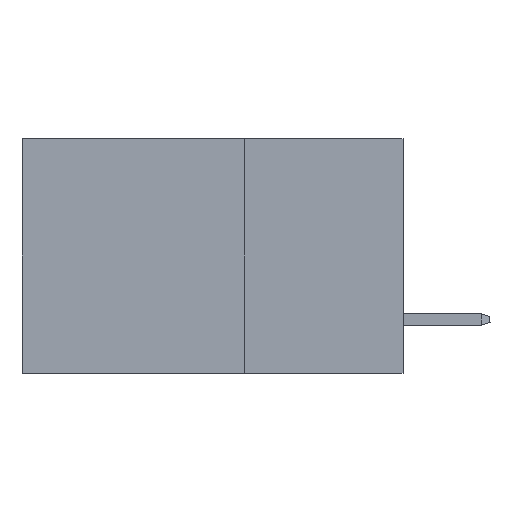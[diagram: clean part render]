
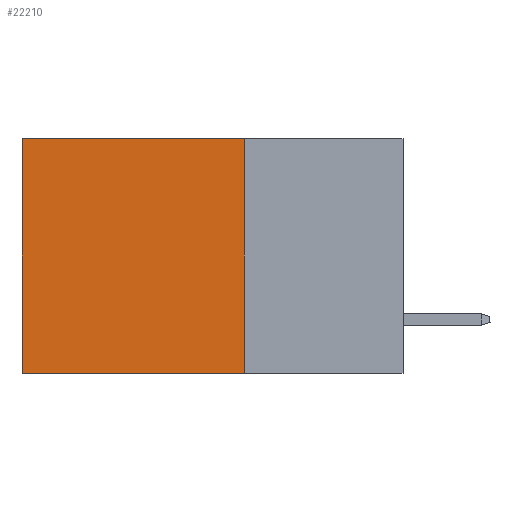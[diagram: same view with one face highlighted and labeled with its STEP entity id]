
A CAD part, left-side view. The second image highlights one B-rep face of the part: STEP entity #22210.
In plain terms, the highlighted planar face has unit normal (-1, 0, 0).
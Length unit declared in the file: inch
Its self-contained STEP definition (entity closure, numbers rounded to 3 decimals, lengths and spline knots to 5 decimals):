
#967 = DIRECTION ( 'NONE',  ( 0., 1., 0. ) ) ;
#1130 = EDGE_CURVE ( 'NONE', #6470, #13392, #18044, .T. ) ;
#1162 = CARTESIAN_POINT ( 'NONE',  ( 0.2875, 0.25, -0.37 ) ) ;
#1659 = CARTESIAN_POINT ( 'NONE',  ( 0.2875, 0.25, -0.37 ) ) ;
#2454 = VERTEX_POINT ( 'NONE', #1659 ) ;
#2565 = ORIENTED_EDGE ( 'NONE', *, *, #24105, .T. ) ;
#3547 = AXIS2_PLACEMENT_3D ( 'NONE', #9867, #39297, #10278 ) ;
#4322 = CARTESIAN_POINT ( 'NONE',  ( 0.2875, 0.25, 0. ) ) ;
#4441 = LINE ( 'NONE', #20441, #12994 ) ;
#4744 = VECTOR ( 'NONE', #10909, 39.37008 ) ;
#6132 = EDGE_LOOP ( 'NONE', ( #20596, #29836, #34292, #2565 ) ) ;
#6470 = VERTEX_POINT ( 'NONE', #37804 ) ;
#7472 = DIRECTION ( 'NONE',  ( 0., 1., 0. ) ) ;
#9821 = EDGE_CURVE ( 'NONE', #29669, #2454, #4441, .T. ) ;
#9867 = CARTESIAN_POINT ( 'NONE',  ( 0.2875, 0.25, 0. ) ) ;
#10278 = DIRECTION ( 'NONE',  ( 0., 0., -1. ) ) ;
#10909 = DIRECTION ( 'NONE',  ( 0., 0., -1. ) ) ;
#12268 = VECTOR ( 'NONE', #7472, 39.37008 ) ;
#12994 = VECTOR ( 'NONE', #30110, 39.37008 ) ;
#13392 = VERTEX_POINT ( 'NONE', #24542 ) ;
#17405 = CARTESIAN_POINT ( 'NONE',  ( 0.2875, 0.25, 0. ) ) ;
#18044 = LINE ( 'NONE', #37199, #4744 ) ;
#20441 = CARTESIAN_POINT ( 'NONE',  ( 0.2875, 0.25, 0. ) ) ;
#20596 = ORIENTED_EDGE ( 'NONE', *, *, #1130, .T. ) ;
#21092 = VECTOR ( 'NONE', #967, 39.37008 ) ;
#22210 = ADVANCED_FACE ( 'NONE', ( #35292 ), #32564, .F. ) ;
#22814 = EDGE_CURVE ( 'NONE', #2454, #13392, #30601, .T. ) ;
#24105 = EDGE_CURVE ( 'NONE', #29669, #6470, #27260, .T. ) ;
#24542 = CARTESIAN_POINT ( 'NONE',  ( 0.2875, 0.6, -0.37 ) ) ;
#27260 = LINE ( 'NONE', #4322, #21092 ) ;
#29669 = VERTEX_POINT ( 'NONE', #17405 ) ;
#29836 = ORIENTED_EDGE ( 'NONE', *, *, #22814, .F. ) ;
#30110 = DIRECTION ( 'NONE',  ( 0., 0., -1. ) ) ;
#30601 = LINE ( 'NONE', #1162, #12268 ) ;
#32564 = PLANE ( 'NONE',  #3547 ) ;
#34292 = ORIENTED_EDGE ( 'NONE', *, *, #9821, .F. ) ;
#35292 = FACE_OUTER_BOUND ( 'NONE', #6132, .T. ) ;
#37199 = CARTESIAN_POINT ( 'NONE',  ( 0.2875, 0.6, 0. ) ) ;
#37804 = CARTESIAN_POINT ( 'NONE',  ( 0.2875, 0.6, 0. ) ) ;
#39297 = DIRECTION ( 'NONE',  ( 1., 0., 0. ) ) ;
